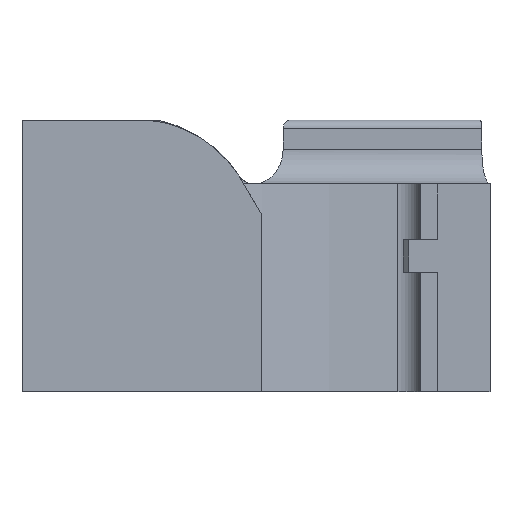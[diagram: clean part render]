
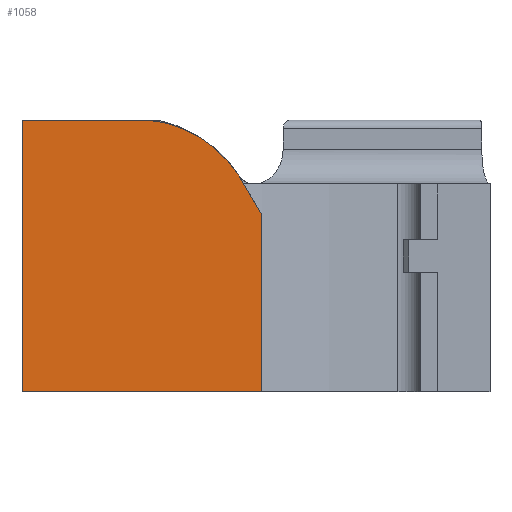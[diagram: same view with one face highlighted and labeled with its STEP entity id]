
A CAD part, front view. The second image highlights one B-rep face of the part: STEP entity #1058.
In plain terms, the highlighted planar face has unit normal (0, -1, 0).
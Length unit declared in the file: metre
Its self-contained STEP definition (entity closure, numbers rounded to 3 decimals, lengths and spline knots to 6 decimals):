
#37=PLANE('',#1182);
#81=FACE_OUTER_BOUND('',#137,.T.);
#137=EDGE_LOOP('',(#881,#882,#883,#884,#885,#886));
#180=LINE('',#1548,#285);
#189=LINE('',#1572,#294);
#198=LINE('',#1606,#303);
#217=LINE('',#1683,#322);
#222=LINE('',#1700,#327);
#285=VECTOR('',#1223,0.01);
#294=VECTOR('',#1244,0.01);
#303=VECTOR('',#1275,0.016179);
#322=VECTOR('',#1338,0.014606);
#327=VECTOR('',#1353,0.01);
#389=CIRCLE('',#1112,0.005582);
#430=VERTEX_POINT('',#1545);
#431=VERTEX_POINT('',#1547);
#433=VERTEX_POINT('',#1553);
#440=VERTEX_POINT('',#1571);
#454=VERTEX_POINT('',#1605);
#490=VERTEX_POINT('',#1681);
#535=EDGE_CURVE('',#431,#430,#180,.T.);
#539=EDGE_CURVE('',#430,#433,#389,.T.);
#547=EDGE_CURVE('',#440,#431,#189,.T.);
#564=EDGE_CURVE('',#454,#440,#198,.T.);
#603=EDGE_CURVE('',#490,#433,#217,.T.);
#610=EDGE_CURVE('',#490,#454,#222,.T.);
#881=ORIENTED_EDGE('',*,*,#610,.T.);
#882=ORIENTED_EDGE('',*,*,#564,.T.);
#883=ORIENTED_EDGE('',*,*,#547,.T.);
#884=ORIENTED_EDGE('',*,*,#535,.T.);
#885=ORIENTED_EDGE('',*,*,#539,.T.);
#886=ORIENTED_EDGE('',*,*,#603,.F.);
#1058=ADVANCED_FACE('',(#81),#37,.F.);
#1112=AXIS2_PLACEMENT_3D('',#1555,#1230,#1231);
#1182=AXIS2_PLACEMENT_3D('',#1824,#1447,#1448);
#1223=DIRECTION('',(-0.505,0.,0.863));
#1230=DIRECTION('center_axis',(0.,-1.,0.));
#1231=DIRECTION('ref_axis',(0.844,0.,0.536));
#1244=DIRECTION('',(0.,0.,1.));
#1275=DIRECTION('',(1.,0.,0.));
#1338=DIRECTION('',(1.,0.,0.));
#1353=DIRECTION('',(0.,0.,-1.));
#1447=DIRECTION('center_axis',(0.,1.,0.));
#1448=DIRECTION('ref_axis',(-1.,0.,0.));
#1545=CARTESIAN_POINT('',(0.014302,-0.00635,0.003058));
#1547=CARTESIAN_POINT('',(0.015312,-0.00635,0.00133));
#1548=CARTESIAN_POINT('',(0.014512,-0.00635,0.002699));
#1553=CARTESIAN_POINT('',(0.010128,-0.00635,0.00562));
#1555=CARTESIAN_POINT('Origin',(0.009592,-0.00635,0.000064));
#1571=CARTESIAN_POINT('',(0.015312,-0.00635,-0.006826));
#1572=CARTESIAN_POINT('',(0.015312,-0.00635,-0.006826));
#1605=CARTESIAN_POINT('',(0.004366,-0.00635,-0.006826));
#1606=CARTESIAN_POINT('',(-0.00605,-0.00635,-0.006826));
#1681=CARTESIAN_POINT('',(0.004366,-0.00635,0.00562));
#1683=CARTESIAN_POINT('',(-0.00605,-0.00635,0.00562));
#1700=CARTESIAN_POINT('',(0.004366,-0.00635,0.00562));
#1824=CARTESIAN_POINT('Origin',(-0.000603,-0.00635,0.00562));
